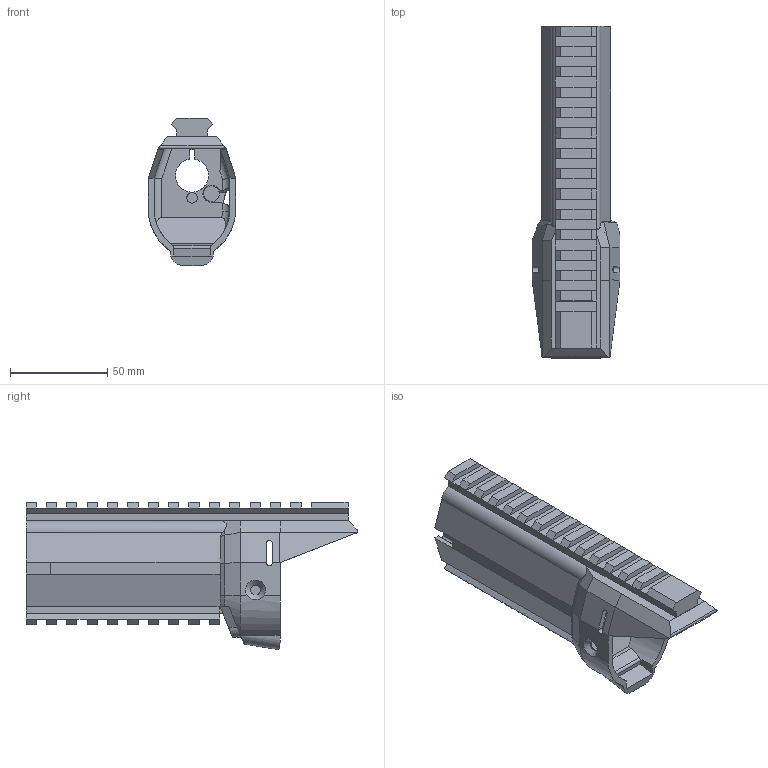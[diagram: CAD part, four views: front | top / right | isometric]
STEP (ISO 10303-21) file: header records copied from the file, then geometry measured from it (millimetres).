
FILE_DESCRIPTION(/* description */ (''),/* implementation_level */ '2;1');
FILE_NAME(/* name */ 'HRR PRA Base v6.step',/* time_stamp */ '2019-12-24T23:32:41-05:00',/* author */ (''),/* organization */ (''),/* preprocessor_version */ 'ST-DEVELOPER v18',/* originating_system */ 'Autodesk Translation Framework v8.12.0.6',/* authorisation */ '');
FILE_SCHEMA (('AUTOMOTIVE_DESIGN { 1 0 10303 214 3 1 1 }'));
Length unit declared in the file: inch
Products named in the file (1): HRR PRA Base
Bounding box: 45 x 170.53 x 75.64 mm (x, y, z)
Volume: 171919.3 mm3; surface area: 59109.8 mm2
Topology: 5 solids, 5 shells, 349 faces, 962 edges, 609 vertices
Faces by surface type: plane 307, cylinder 35, cone 5, bspline 1, torus 1
Full cylindrical faces by diameter (mm): 3 x1, 4.8 x1, 5.207 x1, 5.5 x1
Entity records: 11056 total; most frequent: CARTESIAN_POINT 2118, ORIENTED_EDGE 1924, DIRECTION 1742, EDGE_CURVE 962, LINE 828, VECTOR 828, VERTEX_POINT 609, AXIS2_PLACEMENT_3D 457
